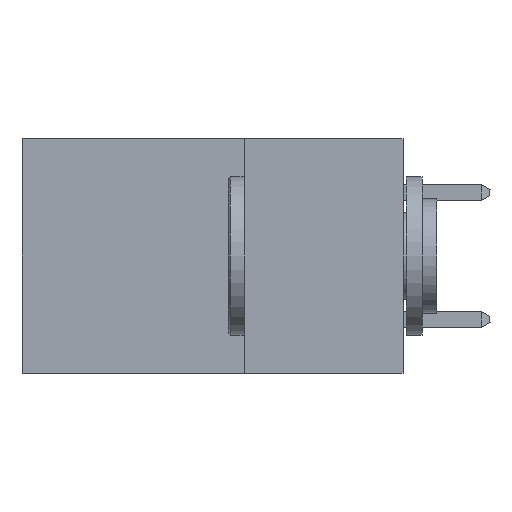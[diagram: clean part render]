
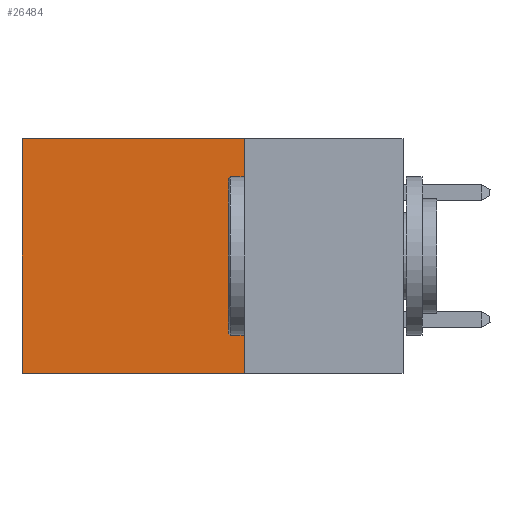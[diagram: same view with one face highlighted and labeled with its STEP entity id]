
A CAD part, left-side view. The second image highlights one B-rep face of the part: STEP entity #26484.
In plain terms, the highlighted planar face has unit normal (-1, 0, 0).
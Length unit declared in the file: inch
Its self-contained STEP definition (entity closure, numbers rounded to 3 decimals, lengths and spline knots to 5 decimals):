
#1531 = VERTEX_POINT ( 'NONE', #6298 ) ;
#1583 = EDGE_LOOP ( 'NONE', ( #6285, #12170, #21868, #27206 ) ) ;
#2920 = EDGE_CURVE ( 'NONE', #30532, #33983, #28543, .T. ) ;
#3397 = DIRECTION ( 'NONE',  ( 0., 0., -1. ) ) ;
#4014 = DIRECTION ( 'NONE',  ( 1., 0., 0. ) ) ;
#6285 = ORIENTED_EDGE ( 'NONE', *, *, #23509, .T. ) ;
#6298 = CARTESIAN_POINT ( 'NONE',  ( 0.2875, 0.6, -0.37 ) ) ;
#6706 = VECTOR ( 'NONE', #12734, 39.37008 ) ;
#7096 = AXIS2_PLACEMENT_3D ( 'NONE', #19360, #4014, #16493 ) ;
#7592 = DIRECTION ( 'NONE',  ( 0., 0., -1. ) ) ;
#8119 = EDGE_CURVE ( 'NONE', #33983, #1531, #25518, .T. ) ;
#8599 = EDGE_CURVE ( 'NONE', #30532, #38565, #17033, .T. ) ;
#12170 = ORIENTED_EDGE ( 'NONE', *, *, #8119, .F. ) ;
#12734 = DIRECTION ( 'NONE',  ( 0., 1., 0. ) ) ;
#14486 = CARTESIAN_POINT ( 'NONE',  ( 0.2875, 0.6, 0. ) ) ;
#15506 = CARTESIAN_POINT ( 'NONE',  ( 0.2875, 0.25, 0. ) ) ;
#16493 = DIRECTION ( 'NONE',  ( 0., 0., -1. ) ) ;
#17033 = LINE ( 'NONE', #36128, #37655 ) ;
#18329 = DIRECTION ( 'NONE',  ( 0., 1., 0. ) ) ;
#19360 = CARTESIAN_POINT ( 'NONE',  ( 0.2875, 0.25, 0. ) ) ;
#20170 = VECTOR ( 'NONE', #3397, 39.37008 ) ;
#21868 = ORIENTED_EDGE ( 'NONE', *, *, #2920, .F. ) ;
#23509 = EDGE_CURVE ( 'NONE', #38565, #1531, #37468, .T. ) ;
#24201 = CARTESIAN_POINT ( 'NONE',  ( 0.2875, 0.25, -0.37 ) ) ;
#25518 = LINE ( 'NONE', #36819, #6706 ) ;
#26484 = ADVANCED_FACE ( 'NONE', ( #36761 ), #28282, .F. ) ;
#27206 = ORIENTED_EDGE ( 'NONE', *, *, #8599, .T. ) ;
#28282 = PLANE ( 'NONE',  #7096 ) ;
#28543 = LINE ( 'NONE', #37572, #32727 ) ;
#30532 = VERTEX_POINT ( 'NONE', #15506 ) ;
#30781 = CARTESIAN_POINT ( 'NONE',  ( 0.2875, 0.6, 0. ) ) ;
#32727 = VECTOR ( 'NONE', #7592, 39.37008 ) ;
#33983 = VERTEX_POINT ( 'NONE', #24201 ) ;
#36128 = CARTESIAN_POINT ( 'NONE',  ( 0.2875, 0.25, 0. ) ) ;
#36761 = FACE_OUTER_BOUND ( 'NONE', #1583, .T. ) ;
#36819 = CARTESIAN_POINT ( 'NONE',  ( 0.2875, 0.25, -0.37 ) ) ;
#37468 = LINE ( 'NONE', #14486, #20170 ) ;
#37572 = CARTESIAN_POINT ( 'NONE',  ( 0.2875, 0.25, 0. ) ) ;
#37655 = VECTOR ( 'NONE', #18329, 39.37008 ) ;
#38565 = VERTEX_POINT ( 'NONE', #30781 ) ;
